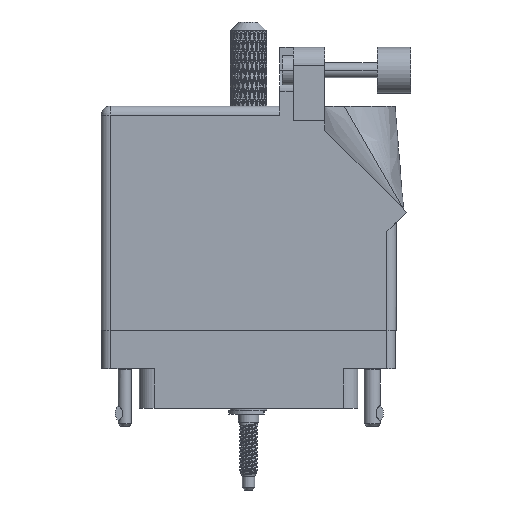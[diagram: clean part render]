
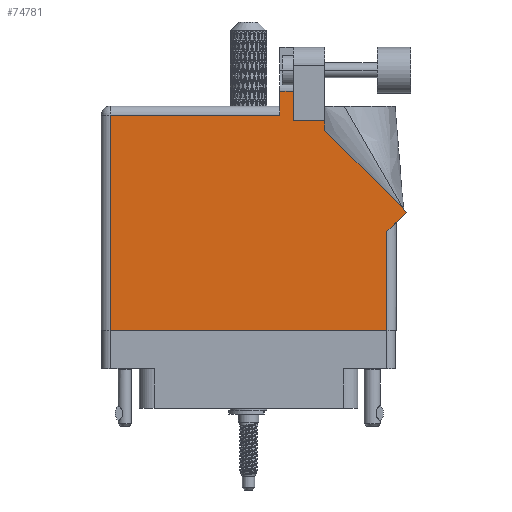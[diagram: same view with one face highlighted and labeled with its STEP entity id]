
A CAD part, front view. The second image highlights one B-rep face of the part: STEP entity #74781.
In plain terms, the highlighted face is planar.
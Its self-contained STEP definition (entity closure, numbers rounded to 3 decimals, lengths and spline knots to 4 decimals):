
#919 = CARTESIAN_POINT ( 'NONE',  ( 2.0807, 0.8077, 0. ) ) ;
#2230 = VERTEX_POINT ( 'NONE', #3358 ) ;
#3358 = CARTESIAN_POINT ( 'NONE',  ( 1.524, 1.3644, 0. ) ) ;
#3363 = VECTOR ( 'NONE', #104447, 39.3701 ) ;
#5348 = CARTESIAN_POINT ( 'NONE',  ( 1.217, 1.6315, 0. ) ) ;
#5859 = EDGE_CURVE ( 'NONE', #66427, #21602, #81885, .T. ) ;
#6203 = CARTESIAN_POINT ( 'NONE',  ( 0., 1.53, 0. ) ) ;
#6342 = DIRECTION ( 'NONE',  ( -1., 0., 0. ) ) ;
#9653 = DIRECTION ( 'NONE',  ( -1., 0., 0. ) ) ;
#11331 = ORIENTED_EDGE ( 'NONE', *, *, #83110, .T. ) ;
#13162 = ORIENTED_EDGE ( 'NONE', *, *, #60801, .T. ) ;
#13629 = VERTEX_POINT ( 'NONE', #104609 ) ;
#14375 = ORIENTED_EDGE ( 'NONE', *, *, #25629, .T. ) ;
#15023 = ORIENTED_EDGE ( 'NONE', *, *, #93851, .T. ) ;
#15269 = CARTESIAN_POINT ( 'NONE',  ( 0.062, 0., 0. ) ) ;
#17184 = CARTESIAN_POINT ( 'NONE',  ( 1.217, 1.468, 0. ) ) ;
#19089 = LINE ( 'NONE', #50227, #48031 ) ;
#19782 = AXIS2_PLACEMENT_3D ( 'NONE', #6203, #72447, #9653 ) ;
#20658 = LINE ( 'NONE', #99697, #64792 ) ;
#21602 = VERTEX_POINT ( 'NONE', #17184 ) ;
#25629 = EDGE_CURVE ( 'NONE', #71877, #78995, #43702, .T. ) ;
#26701 = EDGE_CURVE ( 'NONE', #38707, #109401, #86173, .T. ) ;
#27893 = VECTOR ( 'NONE', #92576, 39.3701 ) ;
#31072 = CARTESIAN_POINT ( 'NONE',  ( 0.062, 1.468, 0. ) ) ;
#32474 = CARTESIAN_POINT ( 'NONE',  ( 2.01, 0.737, 0. ) ) ;
#34751 = CARTESIAN_POINT ( 'NONE',  ( 1.524, 1.43, 0. ) ) ;
#35300 = VECTOR ( 'NONE', #42502, 39.3701 ) ;
#38707 = VERTEX_POINT ( 'NONE', #84285 ) ;
#40415 = DIRECTION ( 'NONE',  ( 1., 0., 0. ) ) ;
#41794 = EDGE_LOOP ( 'NONE', ( #13162, #11331, #109377, #63154, #64304, #64247, #15023, #14375, #49238, #55663, #94149 ) ) ;
#42502 = DIRECTION ( 'NONE',  ( 0., -1., 0. ) ) ;
#43702 = LINE ( 'NONE', #32474, #112789 ) ;
#44104 = CARTESIAN_POINT ( 'NONE',  ( 1.524, 1.3644, 0. ) ) ;
#44442 = LINE ( 'NONE', #65273, #27893 ) ;
#46697 = EDGE_CURVE ( 'NONE', #2230, #75627, #61308, .T. ) ;
#48031 = VECTOR ( 'NONE', #6342, 39.3701 ) ;
#49238 = ORIENTED_EDGE ( 'NONE', *, *, #92382, .T. ) ;
#50227 = CARTESIAN_POINT ( 'NONE',  ( 0., 1.468, 0. ) ) ;
#51193 = PLANE ( 'NONE',  #19782 ) ;
#52803 = CARTESIAN_POINT ( 'NONE',  ( 1.948, 0., 0. ) ) ;
#53521 = LINE ( 'NONE', #59704, #112839 ) ;
#55663 = ORIENTED_EDGE ( 'NONE', *, *, #46697, .T. ) ;
#57708 = VECTOR ( 'NONE', #86449, 39.3701 ) ;
#59704 = CARTESIAN_POINT ( 'NONE',  ( 1.6418, 1.6315, 0. ) ) ;
#60801 = EDGE_CURVE ( 'NONE', #70936, #13629, #44442, .T. ) ;
#61096 = DIRECTION ( 'NONE',  ( -0.707, 0.707, 0. ) ) ;
#61308 = LINE ( 'NONE', #44104, #3363 ) ;
#61339 = CARTESIAN_POINT ( 'NONE',  ( 1.311, 1.43, 0. ) ) ;
#62261 = VERTEX_POINT ( 'NONE', #31072 ) ;
#63154 = ORIENTED_EDGE ( 'NONE', *, *, #93762, .T. ) ;
#63161 = DIRECTION ( 'NONE',  ( -1., 0., 0. ) ) ;
#64247 = ORIENTED_EDGE ( 'NONE', *, *, #26701, .T. ) ;
#64304 = ORIENTED_EDGE ( 'NONE', *, *, #86510, .T. ) ;
#64792 = VECTOR ( 'NONE', #63161, 39.3701 ) ;
#64871 = LINE ( 'NONE', #919, #110300 ) ;
#65273 = CARTESIAN_POINT ( 'NONE',  ( 1.311, 1.43, 0. ) ) ;
#66266 = EDGE_CURVE ( 'NONE', #75627, #70936, #20658, .T. ) ;
#66427 = VERTEX_POINT ( 'NONE', #5348 ) ;
#66754 = VECTOR ( 'NONE', #108904, 39.3701 ) ;
#70936 = VERTEX_POINT ( 'NONE', #61339 ) ;
#71877 = VERTEX_POINT ( 'NONE', #82129 ) ;
#72447 = DIRECTION ( 'NONE',  ( 0., 0., -1. ) ) ;
#74781 = ADVANCED_FACE ( 'NONE', ( #93593 ), #51193, .F. ) ;
#75627 = VERTEX_POINT ( 'NONE', #34751 ) ;
#78995 = VERTEX_POINT ( 'NONE', #91640 ) ;
#81885 = LINE ( 'NONE', #90813, #66754 ) ;
#82129 = CARTESIAN_POINT ( 'NONE',  ( 1.948, 0.675, 0. ) ) ;
#83110 = EDGE_CURVE ( 'NONE', #13629, #66427, #53521, .T. ) ;
#84285 = CARTESIAN_POINT ( 'NONE',  ( 0.062, 0., 0. ) ) ;
#86173 = LINE ( 'NONE', #110580, #112351 ) ;
#86449 = DIRECTION ( 'NONE',  ( 0., 1., 0. ) ) ;
#86510 = EDGE_CURVE ( 'NONE', #62261, #38707, #98655, .T. ) ;
#89391 = LINE ( 'NONE', #103756, #57708 ) ;
#90813 = CARTESIAN_POINT ( 'NONE',  ( 1.217, 1.53, 0. ) ) ;
#91640 = CARTESIAN_POINT ( 'NONE',  ( 2.0807, 0.8077, 0. ) ) ;
#92382 = EDGE_CURVE ( 'NONE', #78995, #2230, #64871, .T. ) ;
#92576 = DIRECTION ( 'NONE',  ( 0., 1., 0. ) ) ;
#93593 = FACE_OUTER_BOUND ( 'NONE', #41794, .T. ) ;
#93762 = EDGE_CURVE ( 'NONE', #21602, #62261, #19089, .T. ) ;
#93851 = EDGE_CURVE ( 'NONE', #109401, #71877, #89391, .T. ) ;
#94149 = ORIENTED_EDGE ( 'NONE', *, *, #66266, .T. ) ;
#94346 = DIRECTION ( 'NONE',  ( -1., 0., 0. ) ) ;
#98655 = LINE ( 'NONE', #15269, #35300 ) ;
#99697 = CARTESIAN_POINT ( 'NONE',  ( 1.524, 1.43, 0. ) ) ;
#102255 = DIRECTION ( 'NONE',  ( 0.707, 0.707, 0. ) ) ;
#103756 = CARTESIAN_POINT ( 'NONE',  ( 1.948, 0.737, 0. ) ) ;
#104447 = DIRECTION ( 'NONE',  ( 0., 1., 0. ) ) ;
#104609 = CARTESIAN_POINT ( 'NONE',  ( 1.311, 1.6315, 0. ) ) ;
#108904 = DIRECTION ( 'NONE',  ( 0., -1., 0. ) ) ;
#109377 = ORIENTED_EDGE ( 'NONE', *, *, #5859, .T. ) ;
#109401 = VERTEX_POINT ( 'NONE', #52803 ) ;
#110300 = VECTOR ( 'NONE', #61096, 39.3701 ) ;
#110580 = CARTESIAN_POINT ( 'NONE',  ( 0., 0., 0. ) ) ;
#112351 = VECTOR ( 'NONE', #40415, 39.3701 ) ;
#112789 = VECTOR ( 'NONE', #102255, 39.3701 ) ;
#112839 = VECTOR ( 'NONE', #94346, 39.3701 ) ;
